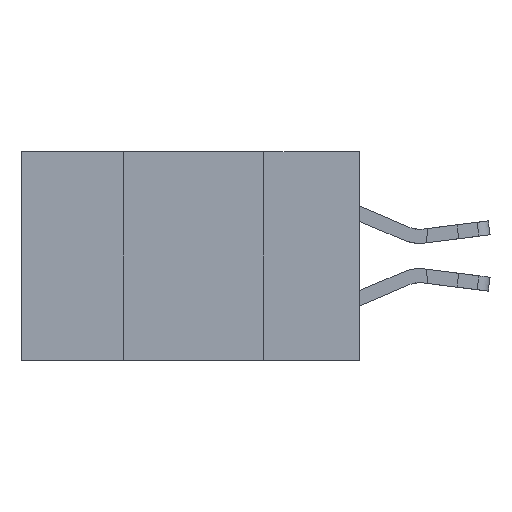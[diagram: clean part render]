
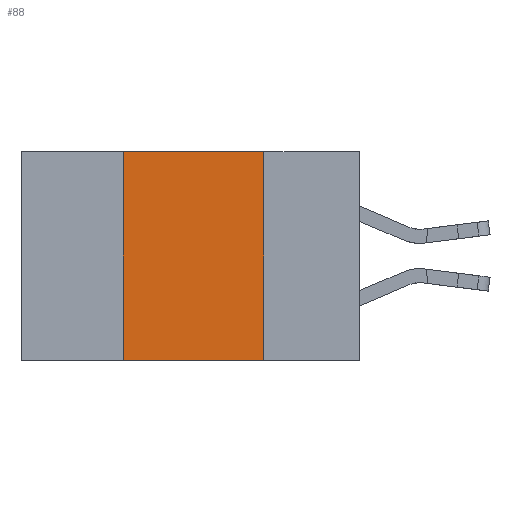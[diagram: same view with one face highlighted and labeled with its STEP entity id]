
A CAD part, left-side view. The second image highlights one B-rep face of the part: STEP entity #88.
In plain terms, the highlighted planar face has unit normal (-1, 0, 0).
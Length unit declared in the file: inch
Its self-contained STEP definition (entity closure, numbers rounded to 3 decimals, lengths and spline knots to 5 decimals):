
#88 = ADVANCED_FACE ( 'NONE', ( #26749 ), #11331, .F. ) ;
#844 = CARTESIAN_POINT ( 'NONE',  ( 0., 0.6, 0. ) ) ;
#1651 = CARTESIAN_POINT ( 'NONE',  ( 0., 0.42, -0.37 ) ) ;
#1873 = DIRECTION ( 'NONE',  ( 1., 0., 0. ) ) ;
#1977 = CARTESIAN_POINT ( 'NONE',  ( 0., 0.6, 0. ) ) ;
#2213 = CARTESIAN_POINT ( 'NONE',  ( 0., 0.17, 0. ) ) ;
#2970 = VERTEX_POINT ( 'NONE', #3092 ) ;
#3092 = CARTESIAN_POINT ( 'NONE',  ( 0., 0.42, 0. ) ) ;
#3301 = ORIENTED_EDGE ( 'NONE', *, *, #28623, .F. ) ;
#4903 = LINE ( 'NONE', #16073, #17603 ) ;
#5146 = CARTESIAN_POINT ( 'NONE',  ( 0., 0.6, -0.37 ) ) ;
#5612 = ORIENTED_EDGE ( 'NONE', *, *, #26794, .F. ) ;
#6885 = AXIS2_PLACEMENT_3D ( 'NONE', #1977, #1873, #18234 ) ;
#8349 = ORIENTED_EDGE ( 'NONE', *, *, #9860, .T. ) ;
#8407 = ORIENTED_EDGE ( 'NONE', *, *, #25522, .F. ) ;
#8950 = DIRECTION ( 'NONE',  ( 0., 0., -1. ) ) ;
#9497 = VECTOR ( 'NONE', #21385, 39.37008 ) ;
#9860 = EDGE_CURVE ( 'NONE', #23142, #26739, #21114, .T. ) ;
#11178 = LINE ( 'NONE', #2213, #28250 ) ;
#11331 = PLANE ( 'NONE',  #6885 ) ;
#11968 = VERTEX_POINT ( 'NONE', #13644 ) ;
#13549 = LINE ( 'NONE', #844, #28811 ) ;
#13644 = CARTESIAN_POINT ( 'NONE',  ( 0., 0.17, 0. ) ) ;
#14680 = DIRECTION ( 'NONE',  ( 0., -1., 0. ) ) ;
#16073 = CARTESIAN_POINT ( 'NONE',  ( 0., 0.42, 0. ) ) ;
#17603 = VECTOR ( 'NONE', #18322, 39.37008 ) ;
#18234 = DIRECTION ( 'NONE',  ( 0., 0., -1. ) ) ;
#18322 = DIRECTION ( 'NONE',  ( 0., 0., 1. ) ) ;
#20662 = CARTESIAN_POINT ( 'NONE',  ( 0., 0.17, -0.37 ) ) ;
#21114 = LINE ( 'NONE', #5146, #9497 ) ;
#21385 = DIRECTION ( 'NONE',  ( 0., -1., 0. ) ) ;
#23142 = VERTEX_POINT ( 'NONE', #1651 ) ;
#25522 = EDGE_CURVE ( 'NONE', #11968, #26739, #11178, .T. ) ;
#25788 = EDGE_LOOP ( 'NONE', ( #8407, #3301, #5612, #8349 ) ) ;
#26739 = VERTEX_POINT ( 'NONE', #20662 ) ;
#26749 = FACE_OUTER_BOUND ( 'NONE', #25788, .T. ) ;
#26794 = EDGE_CURVE ( 'NONE', #23142, #2970, #4903, .T. ) ;
#28250 = VECTOR ( 'NONE', #8950, 39.37008 ) ;
#28623 = EDGE_CURVE ( 'NONE', #2970, #11968, #13549, .T. ) ;
#28811 = VECTOR ( 'NONE', #14680, 39.37008 ) ;
